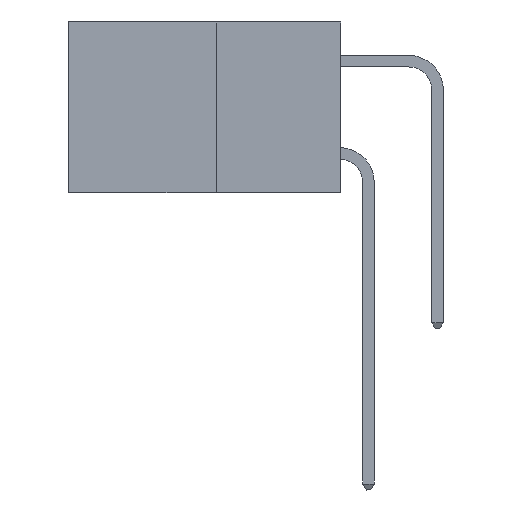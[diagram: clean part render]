
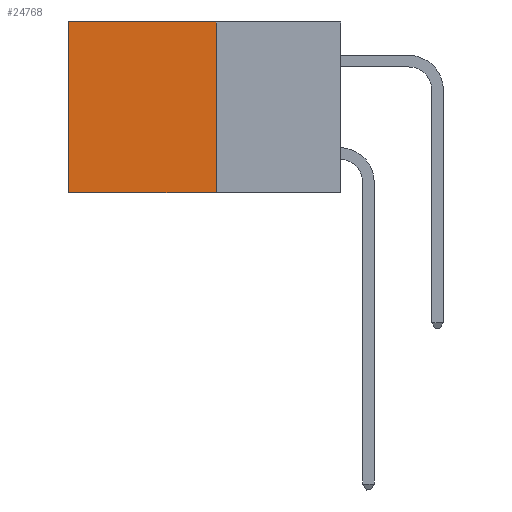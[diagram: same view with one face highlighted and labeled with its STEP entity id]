
A CAD part, left-side view. The second image highlights one B-rep face of the part: STEP entity #24768.
In plain terms, the highlighted planar face has unit normal (-1, 0, 0).
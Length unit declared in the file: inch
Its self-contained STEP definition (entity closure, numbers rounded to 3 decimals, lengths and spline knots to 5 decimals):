
#1085 = EDGE_CURVE ( 'NONE', #2151, #19759, #1543, .T. ) ;
#1543 = LINE ( 'NONE', #2310, #27880 ) ;
#2151 = VERTEX_POINT ( 'NONE', #16498 ) ;
#2310 = CARTESIAN_POINT ( 'NONE',  ( 0.277, 0.27, -0.37 ) ) ;
#2462 = DIRECTION ( 'NONE',  ( 0., 1., 0. ) ) ;
#7770 = LINE ( 'NONE', #11984, #20524 ) ;
#8151 = ORIENTED_EDGE ( 'NONE', *, *, #22320, .T. ) ;
#8222 = VERTEX_POINT ( 'NONE', #10486 ) ;
#9089 = FACE_OUTER_BOUND ( 'NONE', #15349, .T. ) ;
#10325 = VECTOR ( 'NONE', #21207, 39.37008 ) ;
#10341 = ORIENTED_EDGE ( 'NONE', *, *, #24036, .F. ) ;
#10486 = CARTESIAN_POINT ( 'NONE',  ( 0.277, 0.27, 0. ) ) ;
#10545 = CARTESIAN_POINT ( 'NONE',  ( 0.277, 0.27, 0. ) ) ;
#11984 = CARTESIAN_POINT ( 'NONE',  ( 0.277, 0.59, -0.37 ) ) ;
#13021 = VECTOR ( 'NONE', #28292, 39.37008 ) ;
#13825 = LINE ( 'NONE', #10545, #13021 ) ;
#14544 = DIRECTION ( 'NONE',  ( 0., 0., -1. ) ) ;
#15349 = EDGE_LOOP ( 'NONE', ( #8151, #22986, #10341, #20148 ) ) ;
#16230 = CARTESIAN_POINT ( 'NONE',  ( 0.277, 0.27, -0.37 ) ) ;
#16498 = CARTESIAN_POINT ( 'NONE',  ( 0.277, 0.27, -0.37 ) ) ;
#18670 = CARTESIAN_POINT ( 'NONE',  ( 0.277, 0.27, -0.37 ) ) ;
#18776 = VERTEX_POINT ( 'NONE', #25849 ) ;
#18816 = PLANE ( 'NONE',  #26917 ) ;
#19759 = VERTEX_POINT ( 'NONE', #21711 ) ;
#20148 = ORIENTED_EDGE ( 'NONE', *, *, #21916, .T. ) ;
#20524 = VECTOR ( 'NONE', #14544, 39.37008 ) ;
#21207 = DIRECTION ( 'NONE',  ( 0., 0., -1. ) ) ;
#21348 = DIRECTION ( 'NONE',  ( 0., 0., -1. ) ) ;
#21711 = CARTESIAN_POINT ( 'NONE',  ( 0.277, 0.59, -0.37 ) ) ;
#21916 = EDGE_CURVE ( 'NONE', #8222, #18776, #13825, .T. ) ;
#22320 = EDGE_CURVE ( 'NONE', #18776, #19759, #7770, .T. ) ;
#22986 = ORIENTED_EDGE ( 'NONE', *, *, #1085, .F. ) ;
#24036 = EDGE_CURVE ( 'NONE', #8222, #2151, #30577, .T. ) ;
#24768 = ADVANCED_FACE ( 'NONE', ( #9089 ), #18816, .F. ) ;
#25849 = CARTESIAN_POINT ( 'NONE',  ( 0.277, 0.59, 0. ) ) ;
#26917 = AXIS2_PLACEMENT_3D ( 'NONE', #16230, #28882, #21348 ) ;
#27880 = VECTOR ( 'NONE', #2462, 39.37008 ) ;
#28292 = DIRECTION ( 'NONE',  ( 0., 1., 0. ) ) ;
#28882 = DIRECTION ( 'NONE',  ( 1., 0., 0. ) ) ;
#30577 = LINE ( 'NONE', #18670, #10325 ) ;
